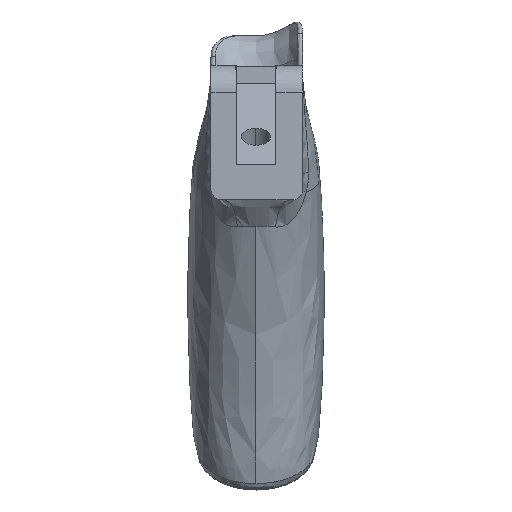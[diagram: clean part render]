
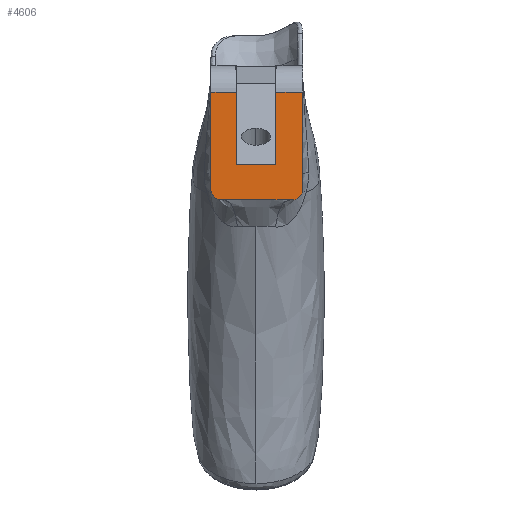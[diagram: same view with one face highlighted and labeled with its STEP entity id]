
A CAD part, top view. The second image highlights one B-rep face of the part: STEP entity #4606.
In plain terms, the highlighted planar face has unit normal (0, 0, 1).
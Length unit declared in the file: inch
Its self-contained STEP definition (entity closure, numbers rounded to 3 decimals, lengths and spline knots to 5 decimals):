
#21 = VECTOR ( 'NONE', #5208, 39.37008 ) ;
#28 = VECTOR ( 'NONE', #5301, 39.37008 ) ;
#118 = CARTESIAN_POINT ( 'NONE',  ( 0.345, -1.2789, 0. ) ) ;
#133 = PLANE ( 'NONE',  #4781 ) ;
#213 = CARTESIAN_POINT ( 'NONE',  ( -0.43, -0.25, 0. ) ) ;
#289 = CARTESIAN_POINT ( 'NONE',  ( -0.43, -1.1789, 0. ) ) ;
#437 = DIRECTION ( 'NONE',  ( 0., -1., 0. ) ) ;
#449 = ORIENTED_EDGE ( 'NONE', *, *, #1822, .T. ) ;
#513 = LINE ( 'NONE', #2123, #28 ) ;
#642 = CARTESIAN_POINT ( 'NONE',  ( -0.43, -0.25, 0. ) ) ;
#690 = VERTEX_POINT ( 'NONE', #1083 ) ;
#821 = CARTESIAN_POINT ( 'NONE',  ( -0.33, -1.2789, 0. ) ) ;
#927 = VECTOR ( 'NONE', #4939, 39.37008 ) ;
#1083 = CARTESIAN_POINT ( 'NONE',  ( 0.1875, -0.25, 0. ) ) ;
#1194 = CARTESIAN_POINT ( 'NONE',  ( -0.43, -1.2789, 0. ) ) ;
#1237 = EDGE_CURVE ( 'NONE', #3900, #4615, #5744, .T. ) ;
#1246 = CARTESIAN_POINT ( 'NONE',  ( -0.43, -1.1789, 0. ) ) ;
#1280 = ORIENTED_EDGE ( 'NONE', *, *, #5531, .T. ) ;
#1289 = VECTOR ( 'NONE', #4006, 39.37008 ) ;
#1527 = LINE ( 'NONE', #1604, #927 ) ;
#1548 = ORIENTED_EDGE ( 'NONE', *, *, #6983, .F. ) ;
#1573 = LINE ( 'NONE', #6498, #6040 ) ;
#1604 = CARTESIAN_POINT ( 'NONE',  ( -0.43, -0.25, 0. ) ) ;
#1665 = EDGE_CURVE ( 'NONE', #1911, #4082, #1573, .T. ) ;
#1687 = DIRECTION ( 'NONE',  ( 1., 0., 0. ) ) ;
#1822 = EDGE_CURVE ( 'NONE', #6395, #3693, #5872, .T. ) ;
#1887 = VERTEX_POINT ( 'NONE', #5865 ) ;
#1893 = CARTESIAN_POINT ( 'NONE',  ( -0.43, -1.2789, 0. ) ) ;
#1910 =( BOUNDED_CURVE ( )  B_SPLINE_CURVE ( 2, ( #289, #1893, #821 ),
 .UNSPECIFIED., .F., .F. ) 
 B_SPLINE_CURVE_WITH_KNOTS ( ( 3, 3 ),
 ( 0., 0.00397 ),
 .UNSPECIFIED. ) 
 CURVE ( )  GEOMETRIC_REPRESENTATION_ITEM ( )  RATIONAL_B_SPLINE_CURVE ( ( 1., 0.707, 1. ) ) 
 REPRESENTATION_ITEM ( '' )  );
#1911 = VERTEX_POINT ( 'NONE', #6908 ) ;
#2123 = CARTESIAN_POINT ( 'NONE',  ( -0.1875, -0.94, 0. ) ) ;
#2252 = FACE_OUTER_BOUND ( 'NONE', #4666, .T. ) ;
#2481 = ORIENTED_EDGE ( 'NONE', *, *, #5279, .F. ) ;
#2517 = CARTESIAN_POINT ( 'NONE',  ( -0.43, -0.25, 0. ) ) ;
#2815 = CARTESIAN_POINT ( 'NONE',  ( -0.1875, -0.25, 0. ) ) ;
#2911 = CARTESIAN_POINT ( 'NONE',  ( -0.1875, 0., 0. ) ) ;
#2927 = EDGE_CURVE ( 'NONE', #3900, #3545, #1527, .T. ) ;
#2973 = VECTOR ( 'NONE', #1687, 39.37008 ) ;
#3219 = LINE ( 'NONE', #5304, #5481 ) ;
#3238 = DIRECTION ( 'NONE',  ( 0., -1., 0. ) ) ;
#3408 = ORIENTED_EDGE ( 'NONE', *, *, #2927, .T. ) ;
#3486 = DIRECTION ( 'NONE',  ( 1., 0., 0. ) ) ;
#3509 = LINE ( 'NONE', #2911, #1289 ) ;
#3545 = VERTEX_POINT ( 'NONE', #1246 ) ;
#3611 = CARTESIAN_POINT ( 'NONE',  ( 0.345, -1.2789, 0. ) ) ;
#3693 = VERTEX_POINT ( 'NONE', #118 ) ;
#3770 = CARTESIAN_POINT ( 'NONE',  ( 0.1875, -0.94, 0. ) ) ;
#3900 = VERTEX_POINT ( 'NONE', #642 ) ;
#4006 = DIRECTION ( 'NONE',  ( 0., -1., 0. ) ) ;
#4082 = VERTEX_POINT ( 'NONE', #7055 ) ;
#4103 = ORIENTED_EDGE ( 'NONE', *, *, #6084, .T. ) ;
#4559 = VERTEX_POINT ( 'NONE', #3770 ) ;
#4606 = ADVANCED_FACE ( 'NONE', ( #2252 ), #133, .T. ) ;
#4615 = VERTEX_POINT ( 'NONE', #2815 ) ;
#4666 = EDGE_LOOP ( 'NONE', ( #449, #6085, #4740, #6437, #4103, #2481, #1548, #5317, #3408, #1280 ) ) ;
#4740 = ORIENTED_EDGE ( 'NONE', *, *, #1665, .F. ) ;
#4781 = AXIS2_PLACEMENT_3D ( 'NONE', #5471, #4936, #3238 ) ;
#4803 = DIRECTION ( 'NONE',  ( 0., -1., 0. ) ) ;
#4830 = CARTESIAN_POINT ( 'NONE',  ( -0.33, -1.2789, 0. ) ) ;
#4936 = DIRECTION ( 'NONE',  ( 0., 0., 1. ) ) ;
#4939 = DIRECTION ( 'NONE',  ( 0., -1., 0. ) ) ;
#5181 = LINE ( 'NONE', #213, #6172 ) ;
#5206 = CARTESIAN_POINT ( 'NONE',  ( 0.445, -1.1789, 0. ) ) ;
#5208 = DIRECTION ( 'NONE',  ( 1., 0., 0. ) ) ;
#5279 = EDGE_CURVE ( 'NONE', #1887, #4559, #513, .T. ) ;
#5301 = DIRECTION ( 'NONE',  ( 1., 0., 0. ) ) ;
#5304 = CARTESIAN_POINT ( 'NONE',  ( 0.1875, 0., 0. ) ) ;
#5317 = ORIENTED_EDGE ( 'NONE', *, *, #1237, .F. ) ;
#5461 =( BOUNDED_CURVE ( )  B_SPLINE_CURVE ( 2, ( #3611, #6254, #5206 ),
 .UNSPECIFIED., .F., .T. ) 
 B_SPLINE_CURVE_WITH_KNOTS ( ( 3, 3 ),
 ( 0., 0.00397 ),
 .UNSPECIFIED. ) 
 CURVE ( )  GEOMETRIC_REPRESENTATION_ITEM ( )  RATIONAL_B_SPLINE_CURVE ( ( 1., 0.707, 1. ) ) 
 REPRESENTATION_ITEM ( '' )  );
#5471 = CARTESIAN_POINT ( 'NONE',  ( -0.43, -0.25, 0. ) ) ;
#5481 = VECTOR ( 'NONE', #437, 39.37008 ) ;
#5531 = EDGE_CURVE ( 'NONE', #3545, #6395, #1910, .T. ) ;
#5744 = LINE ( 'NONE', #2517, #21 ) ;
#5865 = CARTESIAN_POINT ( 'NONE',  ( -0.1875, -0.94, 0. ) ) ;
#5872 = LINE ( 'NONE', #1194, #2973 ) ;
#6040 = VECTOR ( 'NONE', #4803, 39.37008 ) ;
#6084 = EDGE_CURVE ( 'NONE', #690, #4559, #3219, .T. ) ;
#6085 = ORIENTED_EDGE ( 'NONE', *, *, #6819, .T. ) ;
#6144 = EDGE_CURVE ( 'NONE', #690, #1911, #5181, .T. ) ;
#6172 = VECTOR ( 'NONE', #3486, 39.37008 ) ;
#6254 = CARTESIAN_POINT ( 'NONE',  ( 0.445, -1.2789, 0. ) ) ;
#6395 = VERTEX_POINT ( 'NONE', #4830 ) ;
#6437 = ORIENTED_EDGE ( 'NONE', *, *, #6144, .F. ) ;
#6498 = CARTESIAN_POINT ( 'NONE',  ( 0.445, -0.25, 0. ) ) ;
#6819 = EDGE_CURVE ( 'NONE', #3693, #4082, #5461, .T. ) ;
#6908 = CARTESIAN_POINT ( 'NONE',  ( 0.445, -0.25, 0. ) ) ;
#6983 = EDGE_CURVE ( 'NONE', #4615, #1887, #3509, .T. ) ;
#7055 = CARTESIAN_POINT ( 'NONE',  ( 0.445, -1.1789, 0. ) ) ;
